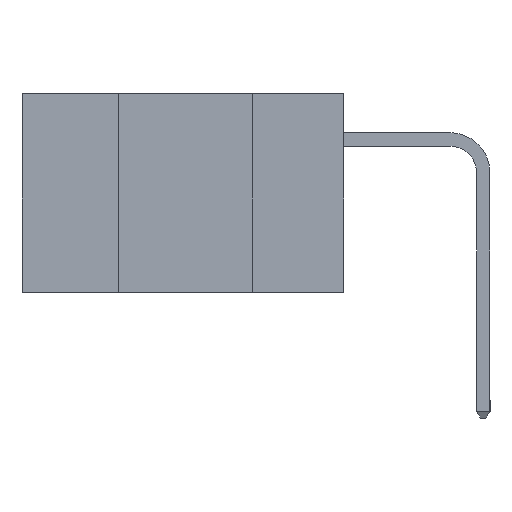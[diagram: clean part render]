
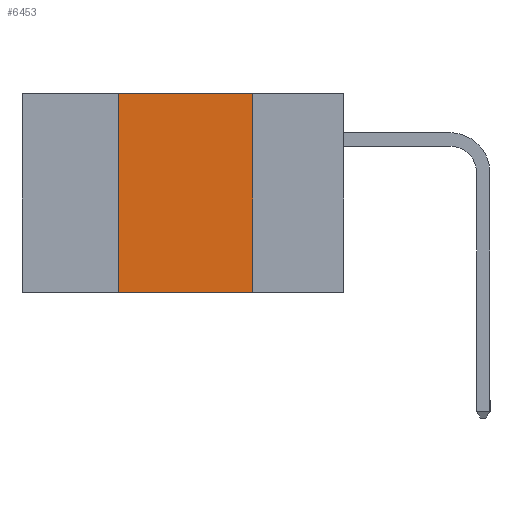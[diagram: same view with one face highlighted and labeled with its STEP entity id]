
A CAD part, left-side view. The second image highlights one B-rep face of the part: STEP entity #6453.
In plain terms, the highlighted planar face has unit normal (-1, 0, 0).
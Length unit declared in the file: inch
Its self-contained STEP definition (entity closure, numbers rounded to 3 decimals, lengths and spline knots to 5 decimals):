
#67 = CARTESIAN_POINT ( 'NONE',  ( 0., 0.17, 0. ) ) ;
#423 = ORIENTED_EDGE ( 'NONE', *, *, #1878, .F. ) ;
#814 = CARTESIAN_POINT ( 'NONE',  ( 0., 0.6, 0. ) ) ;
#1470 = DIRECTION ( 'NONE',  ( 0., -1., 0. ) ) ;
#1878 = EDGE_CURVE ( 'NONE', #6124, #9276, #19512, .T. ) ;
#2263 = CARTESIAN_POINT ( 'NONE',  ( 0., 0.42, -0.37 ) ) ;
#3627 = EDGE_LOOP ( 'NONE', ( #423, #6804, #5578, #14035 ) ) ;
#3758 = CARTESIAN_POINT ( 'NONE',  ( 0., 0.17, -0.37 ) ) ;
#4156 = VECTOR ( 'NONE', #1470, 39.37008 ) ;
#4246 = LINE ( 'NONE', #5180, #20008 ) ;
#5170 = VERTEX_POINT ( 'NONE', #2263 ) ;
#5180 = CARTESIAN_POINT ( 'NONE',  ( 0., 0.42, -0.37 ) ) ;
#5183 = DIRECTION ( 'NONE',  ( 0., -1., 0. ) ) ;
#5433 = EDGE_CURVE ( 'NONE', #5170, #9276, #15340, .T. ) ;
#5578 = ORIENTED_EDGE ( 'NONE', *, *, #8609, .F. ) ;
#6124 = VERTEX_POINT ( 'NONE', #67 ) ;
#6453 = ADVANCED_FACE ( 'NONE', ( #12803 ), #8725, .F. ) ;
#6804 = ORIENTED_EDGE ( 'NONE', *, *, #12889, .F. ) ;
#7880 = CARTESIAN_POINT ( 'NONE',  ( 0., 0.17, -0.37 ) ) ;
#7924 = CARTESIAN_POINT ( 'NONE',  ( 0., 0.42, 0. ) ) ;
#8609 = EDGE_CURVE ( 'NONE', #5170, #17002, #4246, .T. ) ;
#8646 = DIRECTION ( 'NONE',  ( 0., 0., -1. ) ) ;
#8725 = PLANE ( 'NONE',  #10481 ) ;
#9276 = VERTEX_POINT ( 'NONE', #3758 ) ;
#9284 = VECTOR ( 'NONE', #5183, 39.37008 ) ;
#10342 = DIRECTION ( 'NONE',  ( 0., 0., -1. ) ) ;
#10481 = AXIS2_PLACEMENT_3D ( 'NONE', #814, #19730, #10342 ) ;
#12803 = FACE_OUTER_BOUND ( 'NONE', #3627, .T. ) ;
#12889 = EDGE_CURVE ( 'NONE', #17002, #6124, #13064, .T. ) ;
#13064 = LINE ( 'NONE', #16303, #9284 ) ;
#13178 = DIRECTION ( 'NONE',  ( 0., 0., 1. ) ) ;
#14035 = ORIENTED_EDGE ( 'NONE', *, *, #5433, .T. ) ;
#15340 = LINE ( 'NONE', #15724, #4156 ) ;
#15724 = CARTESIAN_POINT ( 'NONE',  ( 0., 0.6, -0.37 ) ) ;
#16303 = CARTESIAN_POINT ( 'NONE',  ( 0., 0.6, 0. ) ) ;
#17002 = VERTEX_POINT ( 'NONE', #7924 ) ;
#19049 = VECTOR ( 'NONE', #8646, 39.37008 ) ;
#19512 = LINE ( 'NONE', #7880, #19049 ) ;
#19730 = DIRECTION ( 'NONE',  ( 1., 0., 0. ) ) ;
#20008 = VECTOR ( 'NONE', #13178, 39.37008 ) ;
